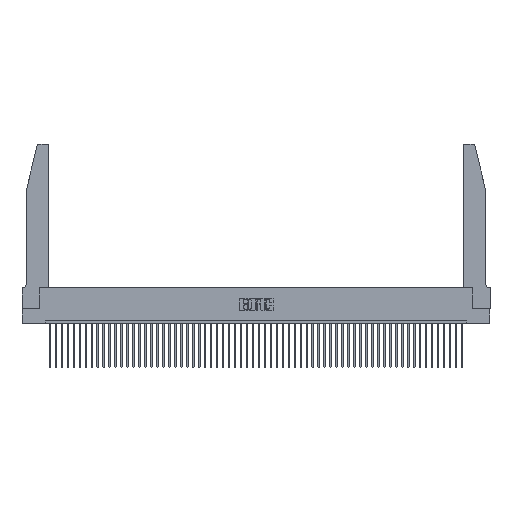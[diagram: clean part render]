
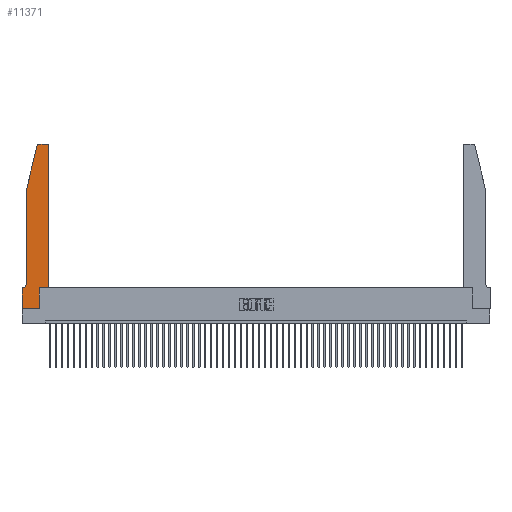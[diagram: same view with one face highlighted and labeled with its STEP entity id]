
A CAD part, top view. The second image highlights one B-rep face of the part: STEP entity #11371.
In plain terms, the highlighted planar face has unit normal (0, 0, 1).
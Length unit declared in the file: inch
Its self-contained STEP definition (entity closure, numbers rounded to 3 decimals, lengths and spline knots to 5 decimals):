
#1693 = CARTESIAN_POINT ( 'NONE',  ( 0.0755, 0.35, 0.37 ) ) ;
#1840 = CARTESIAN_POINT ( 'NONE',  ( 0.4505, 0.35, 0.37 ) ) ;
#2182 = CARTESIAN_POINT ( 'NONE',  ( 0.0755, 0.42, 0.37 ) ) ;
#2548 = LINE ( 'NONE', #43414, #19483 ) ;
#2559 = CARTESIAN_POINT ( 'NONE',  ( 0.2865, 0., 0.37 ) ) ;
#3255 = DIRECTION ( 'NONE',  ( 0., 1., 0. ) ) ;
#3574 = EDGE_CURVE ( 'NONE', #29966, #41736, #21873, .T. ) ;
#3716 = LINE ( 'NONE', #1840, #23143 ) ;
#4033 = AXIS2_PLACEMENT_3D ( 'NONE', #24449, #28633, #20595 ) ;
#4074 = VECTOR ( 'NONE', #24104, 39.37008 ) ;
#4680 = CIRCLE ( 'NONE', #50366, 0.07 ) ;
#5769 = DIRECTION ( 'NONE',  ( -1., 0., 0. ) ) ;
#5864 = EDGE_CURVE ( 'NONE', #22029, #39205, #39435, .T. ) ;
#6071 = VERTEX_POINT ( 'NONE', #44166 ) ;
#6244 = LINE ( 'NONE', #27994, #47738 ) ;
#6767 = ORIENTED_EDGE ( 'NONE', *, *, #49701, .T. ) ;
#6902 = VERTEX_POINT ( 'NONE', #14941 ) ;
#7487 = VECTOR ( 'NONE', #21559, 39.37008 ) ;
#7566 = EDGE_CURVE ( 'NONE', #41736, #43765, #26028, .T. ) ;
#8701 = CARTESIAN_POINT ( 'NONE',  ( 0.0755, 2., 0.37 ) ) ;
#9860 = ORIENTED_EDGE ( 'NONE', *, *, #10720, .T. ) ;
#10029 = CARTESIAN_POINT ( 'NONE',  ( 0., 0.35, 0.37 ) ) ;
#10084 = DIRECTION ( 'NONE',  ( 0., 1., 0. ) ) ;
#10435 = CARTESIAN_POINT ( 'NONE',  ( 0.2605, 2.75, 0.37 ) ) ;
#10720 = EDGE_CURVE ( 'NONE', #6902, #29966, #3716, .T. ) ;
#10981 = VERTEX_POINT ( 'NONE', #18964 ) ;
#11371 = ADVANCED_FACE ( 'NONE', ( #43118 ), #46695, .T. ) ;
#12085 = ORIENTED_EDGE ( 'NONE', *, *, #7566, .T. ) ;
#12727 = EDGE_CURVE ( 'NONE', #39205, #32362, #19646, .T. ) ;
#12910 = ORIENTED_EDGE ( 'NONE', *, *, #16183, .T. ) ;
#14701 = CARTESIAN_POINT ( 'NONE',  ( 0.284, 2.72, 0.37 ) ) ;
#14941 = CARTESIAN_POINT ( 'NONE',  ( 0.4505, 0.35, 0.37 ) ) ;
#15675 = VERTEX_POINT ( 'NONE', #2182 ) ;
#15753 = CARTESIAN_POINT ( 'NONE',  ( 0.0055, 0.42, 0.37 ) ) ;
#15962 = CARTESIAN_POINT ( 'NONE',  ( 0.2865, 0.35, 0.37 ) ) ;
#16149 = AXIS2_PLACEMENT_3D ( 'NONE', #38248, #21540, #42933 ) ;
#16183 = EDGE_CURVE ( 'NONE', #42403, #25294, #49752, .T. ) ;
#16358 = ORIENTED_EDGE ( 'NONE', *, *, #5864, .T. ) ;
#17341 = ORIENTED_EDGE ( 'NONE', *, *, #51159, .T. ) ;
#18964 = CARTESIAN_POINT ( 'NONE',  ( 0.25487, 2.72718, 0.37 ) ) ;
#19382 = DIRECTION ( 'NONE',  ( 1., 0., 0. ) ) ;
#19483 = VECTOR ( 'NONE', #39074, 39.37008 ) ;
#19646 = LINE ( 'NONE', #15962, #41663 ) ;
#20595 = DIRECTION ( 'NONE',  ( 1., 0., 0. ) ) ;
#20669 = CARTESIAN_POINT ( 'NONE',  ( 0.284, 2.75, 0.37 ) ) ;
#20795 = VECTOR ( 'NONE', #29852, 39.37008 ) ;
#21540 = DIRECTION ( 'NONE',  ( 0., 0., 1. ) ) ;
#21559 = DIRECTION ( 'NONE',  ( 1., 0., 0. ) ) ;
#21873 = CIRCLE ( 'NONE', #4033, 0.03 ) ;
#22029 = VERTEX_POINT ( 'NONE', #52518 ) ;
#23143 = VECTOR ( 'NONE', #10084, 39.37008 ) ;
#23218 = VECTOR ( 'NONE', #30262, 39.37008 ) ;
#23571 = AXIS2_PLACEMENT_3D ( 'NONE', #14701, #48216, #19382 ) ;
#24104 = DIRECTION ( 'NONE',  ( -1., 0., 0. ) ) ;
#24449 = CARTESIAN_POINT ( 'NONE',  ( 0.4205, 2.72, 0.37 ) ) ;
#24837 = ORIENTED_EDGE ( 'NONE', *, *, #47519, .T. ) ;
#25294 = VERTEX_POINT ( 'NONE', #10029 ) ;
#26028 = LINE ( 'NONE', #10435, #4074 ) ;
#26290 = EDGE_CURVE ( 'NONE', #32362, #6902, #34610, .T. ) ;
#26626 = CARTESIAN_POINT ( 'NONE',  ( 0., 0., 0.37 ) ) ;
#27992 = LINE ( 'NONE', #8701, #20795 ) ;
#27994 = CARTESIAN_POINT ( 'NONE',  ( 0.0755, 2., 0.37 ) ) ;
#28633 = DIRECTION ( 'NONE',  ( 0., 0., 1. ) ) ;
#28802 = CARTESIAN_POINT ( 'NONE',  ( 0.4205, 2.75, 0.37 ) ) ;
#29713 = CARTESIAN_POINT ( 'NONE',  ( 0.0055, 0.35, 0.37 ) ) ;
#29852 = DIRECTION ( 'NONE',  ( -0.239, -0.971, 0. ) ) ;
#29966 = VERTEX_POINT ( 'NONE', #51345 ) ;
#30141 = ORIENTED_EDGE ( 'NONE', *, *, #26290, .T. ) ;
#30262 = DIRECTION ( 'NONE',  ( 1., 0., 0. ) ) ;
#32362 = VERTEX_POINT ( 'NONE', #38794 ) ;
#32810 = DIRECTION ( 'NONE',  ( -1., 0., 0. ) ) ;
#33363 = EDGE_CURVE ( 'NONE', #43765, #10981, #40317, .T. ) ;
#34610 = LINE ( 'NONE', #41432, #7487 ) ;
#36107 = DIRECTION ( 'NONE',  ( 0., -1., 0. ) ) ;
#36432 = DIRECTION ( 'NONE',  ( 0., 0., -1. ) ) ;
#38103 = EDGE_LOOP ( 'NONE', ( #12085, #38705, #24837, #51444, #6767, #12910, #17341, #16358, #39142, #30141, #9860, #40364 ) ) ;
#38248 = CARTESIAN_POINT ( 'NONE',  ( 0., 0.35, 0.37 ) ) ;
#38686 = VECTOR ( 'NONE', #5769, 39.37008 ) ;
#38705 = ORIENTED_EDGE ( 'NONE', *, *, #33363, .T. ) ;
#38794 = CARTESIAN_POINT ( 'NONE',  ( 0.2865, 0.35, 0.37 ) ) ;
#39074 = DIRECTION ( 'NONE',  ( 0., -1., 0. ) ) ;
#39142 = ORIENTED_EDGE ( 'NONE', *, *, #12727, .T. ) ;
#39205 = VERTEX_POINT ( 'NONE', #2559 ) ;
#39435 = LINE ( 'NONE', #26626, #23218 ) ;
#40317 = CIRCLE ( 'NONE', #23571, 0.03 ) ;
#40364 = ORIENTED_EDGE ( 'NONE', *, *, #3574, .T. ) ;
#41432 = CARTESIAN_POINT ( 'NONE',  ( 0.4505, 0.35, 0.37 ) ) ;
#41663 = VECTOR ( 'NONE', #3255, 39.37008 ) ;
#41736 = VERTEX_POINT ( 'NONE', #28802 ) ;
#42403 = VERTEX_POINT ( 'NONE', #29713 ) ;
#42933 = DIRECTION ( 'NONE',  ( 1., 0., 0. ) ) ;
#43118 = FACE_OUTER_BOUND ( 'NONE', #38103, .T. ) ;
#43414 = CARTESIAN_POINT ( 'NONE',  ( 0., 0., 0.37 ) ) ;
#43620 = EDGE_CURVE ( 'NONE', #6071, #15675, #6244, .T. ) ;
#43765 = VERTEX_POINT ( 'NONE', #20669 ) ;
#44166 = CARTESIAN_POINT ( 'NONE',  ( 0.0755, 2., 0.37 ) ) ;
#46695 = PLANE ( 'NONE',  #16149 ) ;
#47519 = EDGE_CURVE ( 'NONE', #10981, #6071, #27992, .T. ) ;
#47738 = VECTOR ( 'NONE', #36107, 39.37008 ) ;
#48216 = DIRECTION ( 'NONE',  ( 0., 0., 1. ) ) ;
#49701 = EDGE_CURVE ( 'NONE', #15675, #42403, #4680, .T. ) ;
#49752 = LINE ( 'NONE', #1693, #38686 ) ;
#50366 = AXIS2_PLACEMENT_3D ( 'NONE', #15753, #36432, #32810 ) ;
#51159 = EDGE_CURVE ( 'NONE', #25294, #22029, #2548, .T. ) ;
#51345 = CARTESIAN_POINT ( 'NONE',  ( 0.4505, 2.72, 0.37 ) ) ;
#51444 = ORIENTED_EDGE ( 'NONE', *, *, #43620, .T. ) ;
#52518 = CARTESIAN_POINT ( 'NONE',  ( 0., 0., 0.37 ) ) ;
